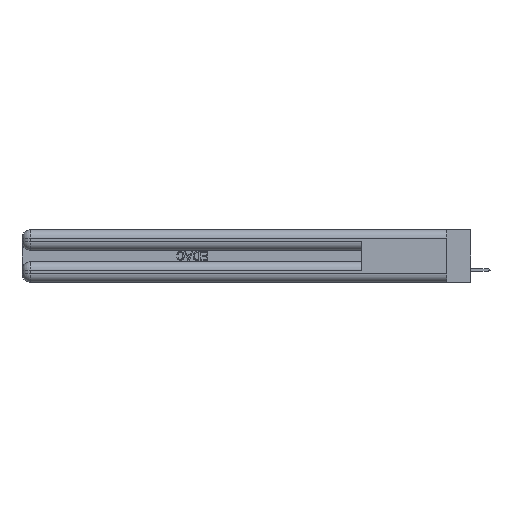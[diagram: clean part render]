
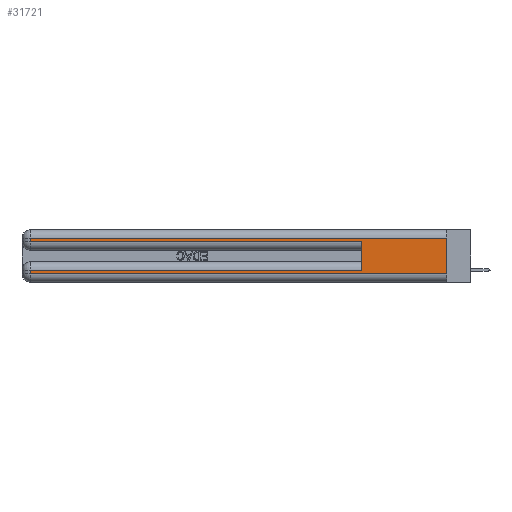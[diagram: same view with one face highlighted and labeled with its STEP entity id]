
A CAD part, left-side view. The second image highlights one B-rep face of the part: STEP entity #31721.
In plain terms, the highlighted planar face has unit normal (-1, 0, 0).
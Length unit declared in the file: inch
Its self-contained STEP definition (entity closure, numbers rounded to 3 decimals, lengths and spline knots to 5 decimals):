
#697 = LINE ( 'NONE', #15663, #35432 ) ;
#828 = LINE ( 'NONE', #12840, #15017 ) ;
#1347 = EDGE_LOOP ( 'NONE', ( #18072, #3329, #24701, #32517, #22834, #19720, #29921, #32556 ) ) ;
#1427 = CARTESIAN_POINT ( 'NONE',  ( 0., 0.6, 0.085 ) ) ;
#3329 = ORIENTED_EDGE ( 'NONE', *, *, #34287, .T. ) ;
#4168 = CARTESIAN_POINT ( 'NONE',  ( 0., 0., 0.085 ) ) ;
#4610 = CARTESIAN_POINT ( 'NONE',  ( 0., 0., 0.37 ) ) ;
#5220 = CARTESIAN_POINT ( 'NONE',  ( 0., 0., 0.31 ) ) ;
#5843 = CARTESIAN_POINT ( 'NONE',  ( 0., 2.94, 0.37 ) ) ;
#6118 = EDGE_CURVE ( 'NONE', #38293, #37200, #13019, .T. ) ;
#6209 = EDGE_CURVE ( 'NONE', #24142, #33460, #7916, .T. ) ;
#6368 = VERTEX_POINT ( 'NONE', #12394 ) ;
#7720 = CARTESIAN_POINT ( 'NONE',  ( 0., 0., 0.37 ) ) ;
#7916 = LINE ( 'NONE', #7720, #8010 ) ;
#8010 = VECTOR ( 'NONE', #11063, 39.37008 ) ;
#10326 = CARTESIAN_POINT ( 'NONE',  ( 0., 0., 0.31 ) ) ;
#11063 = DIRECTION ( 'NONE',  ( 0., 0., -1. ) ) ;
#11072 = CARTESIAN_POINT ( 'NONE',  ( 0., 2.94, 0.085 ) ) ;
#12394 = CARTESIAN_POINT ( 'NONE',  ( 0., 2.94, 0.285 ) ) ;
#12840 = CARTESIAN_POINT ( 'NONE',  ( 0., 0.6, 0.145 ) ) ;
#13019 = LINE ( 'NONE', #4168, #31210 ) ;
#13723 = LINE ( 'NONE', #37295, #13817 ) ;
#13817 = VECTOR ( 'NONE', #28448, 39.37008 ) ;
#14745 = EDGE_CURVE ( 'NONE', #6368, #19948, #37898, .T. ) ;
#15017 = VECTOR ( 'NONE', #36809, 39.37008 ) ;
#15663 = CARTESIAN_POINT ( 'NONE',  ( 0., 2.94, 0.37 ) ) ;
#15767 = CARTESIAN_POINT ( 'NONE',  ( 0., 0., 0.285 ) ) ;
#17363 = EDGE_CURVE ( 'NONE', #37200, #22457, #697, .T. ) ;
#17998 = DIRECTION ( 'NONE',  ( 0., 0., -1. ) ) ;
#18072 = ORIENTED_EDGE ( 'NONE', *, *, #6209, .F. ) ;
#19156 = LINE ( 'NONE', #10326, #26785 ) ;
#19720 = ORIENTED_EDGE ( 'NONE', *, *, #6118, .T. ) ;
#19948 = VERTEX_POINT ( 'NONE', #36947 ) ;
#21912 = FACE_OUTER_BOUND ( 'NONE', #1347, .T. ) ;
#22457 = VERTEX_POINT ( 'NONE', #24355 ) ;
#22834 = ORIENTED_EDGE ( 'NONE', *, *, #24507, .F. ) ;
#24142 = VERTEX_POINT ( 'NONE', #5220 ) ;
#24197 = VECTOR ( 'NONE', #17998, 39.37008 ) ;
#24355 = CARTESIAN_POINT ( 'NONE',  ( 0., 2.94, 0.06 ) ) ;
#24507 = EDGE_CURVE ( 'NONE', #38293, #19948, #828, .T. ) ;
#24701 = ORIENTED_EDGE ( 'NONE', *, *, #32745, .T. ) ;
#25014 = DIRECTION ( 'NONE',  ( 0., 1., 0. ) ) ;
#25018 = CARTESIAN_POINT ( 'NONE',  ( 0., 0., 0.06 ) ) ;
#25516 = EDGE_CURVE ( 'NONE', #22457, #33460, #13723, .T. ) ;
#25793 = VECTOR ( 'NONE', #34950, 39.37008 ) ;
#26785 = VECTOR ( 'NONE', #34486, 39.37008 ) ;
#27629 = CARTESIAN_POINT ( 'NONE',  ( 0., 2.94, 0.31 ) ) ;
#28448 = DIRECTION ( 'NONE',  ( 0., -1., 0. ) ) ;
#28575 = PLANE ( 'NONE',  #36131 ) ;
#29921 = ORIENTED_EDGE ( 'NONE', *, *, #17363, .T. ) ;
#30437 = VERTEX_POINT ( 'NONE', #27629 ) ;
#31210 = VECTOR ( 'NONE', #25014, 39.37008 ) ;
#31721 = ADVANCED_FACE ( 'NONE', ( #21912 ), #28575, .F. ) ;
#32517 = ORIENTED_EDGE ( 'NONE', *, *, #14745, .T. ) ;
#32556 = ORIENTED_EDGE ( 'NONE', *, *, #25516, .T. ) ;
#32745 = EDGE_CURVE ( 'NONE', #30437, #6368, #38066, .T. ) ;
#33460 = VERTEX_POINT ( 'NONE', #25018 ) ;
#33900 = DIRECTION ( 'NONE',  ( 0., 0., -1. ) ) ;
#33931 = DIRECTION ( 'NONE',  ( 0., 0., -1. ) ) ;
#34287 = EDGE_CURVE ( 'NONE', #24142, #30437, #19156, .T. ) ;
#34486 = DIRECTION ( 'NONE',  ( 0., 1., 0. ) ) ;
#34950 = DIRECTION ( 'NONE',  ( 0., -1., 0. ) ) ;
#35432 = VECTOR ( 'NONE', #33931, 39.37008 ) ;
#36131 = AXIS2_PLACEMENT_3D ( 'NONE', #4610, #37421, #33900 ) ;
#36809 = DIRECTION ( 'NONE',  ( 0., 0., 1. ) ) ;
#36947 = CARTESIAN_POINT ( 'NONE',  ( 0., 0.6, 0.285 ) ) ;
#37200 = VERTEX_POINT ( 'NONE', #11072 ) ;
#37295 = CARTESIAN_POINT ( 'NONE',  ( 0., 0., 0.06 ) ) ;
#37421 = DIRECTION ( 'NONE',  ( 1., 0., 0. ) ) ;
#37898 = LINE ( 'NONE', #15767, #25793 ) ;
#38066 = LINE ( 'NONE', #5843, #24197 ) ;
#38293 = VERTEX_POINT ( 'NONE', #1427 ) ;
